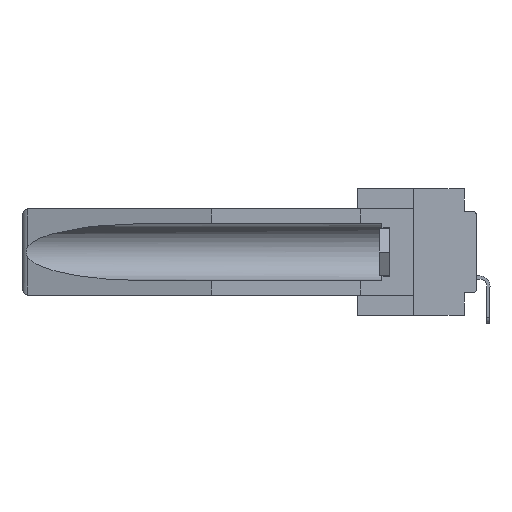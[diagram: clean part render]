
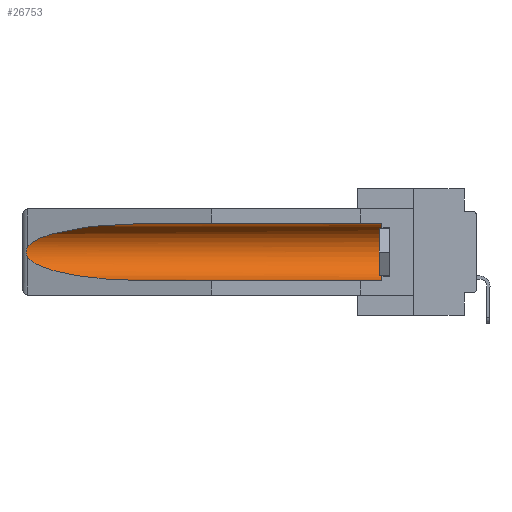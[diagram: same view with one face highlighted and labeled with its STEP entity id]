
A CAD part, left-side view. The second image highlights one B-rep face of the part: STEP entity #26753.
In plain terms, the highlighted cylindrical face has radius 2.857 mm (diameter 5.715 mm), a partial arc.
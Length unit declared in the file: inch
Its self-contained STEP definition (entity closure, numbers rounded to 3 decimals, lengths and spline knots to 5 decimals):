
#281 = VERTEX_POINT ( 'NONE', #3739 ) ;
#1954 = CARTESIAN_POINT ( 'NONE',  ( 0.2675, 1.53308, -0.17534 ) ) ;
#2335 = CARTESIAN_POINT ( 'NONE',  ( 0.2673, 1.53269, -0.17917 ) ) ;
#2608 = AXIS2_PLACEMENT_3D ( 'NONE', #23767, #16681, #25966 ) ;
#3291 = ORIENTED_EDGE ( 'NONE', *, *, #8695, .F. ) ;
#3420 = CARTESIAN_POINT ( 'NONE',  ( 0.26655, 1.53094, -0.18657 ) ) ;
#3661 = EDGE_CURVE ( 'NONE', #20136, #19773, #11870, .T. ) ;
#3739 = CARTESIAN_POINT ( 'NONE',  ( 0.155, 1.07973, -0.059 ) ) ;
#4217 = AXIS2_PLACEMENT_3D ( 'NONE', #11792, #9875, #16605 ) ;
#4889 = FACE_OUTER_BOUND ( 'NONE', #15215, .T. ) ;
#5228 = CARTESIAN_POINT ( 'NONE',  ( 0.2673, 1.5327, -0.16383 ) ) ;
#7863 = CARTESIAN_POINT ( 'NONE',  ( 0.26537, 1.52718, -0.14972 ) ) ;
#8695 = EDGE_CURVE ( 'NONE', #20136, #28436, #20644, .T. ) ;
#9158 = CARTESIAN_POINT ( 'NONE',  ( 0.21114, 1.30732, -0.284 ) ) ;
#9875 = DIRECTION ( 'NONE',  ( 0., 1., 0. ) ) ;
#10264 = CARTESIAN_POINT ( 'NONE',  ( 0.25451, 1.48313, -0.09465 ) ) ;
#11792 = CARTESIAN_POINT ( 'NONE',  ( 0.155, -0.30754, -0.1715 ) ) ;
#11870 = CIRCLE ( 'NONE', #2608, 0.1125 ) ;
#12776 = CARTESIAN_POINT ( 'NONE',  ( 0.155, 1.07973, -0.059 ) ) ;
#13152 = CARTESIAN_POINT ( 'NONE',  ( 0.2675, 1.53308, -0.16763 ) ) ;
#13375 = VECTOR ( 'NONE', #17002, 39.37008 ) ;
#13476 = CARTESIAN_POINT ( 'NONE',  ( 0.26537, 1.52718, -0.14972 ) ) ;
#13770 = CARTESIAN_POINT ( 'NONE',  ( 0.155, 0.126, -0.284 ) ) ;
#14582 = EDGE_CURVE ( 'NONE', #19773, #281, #29049, .T. ) ;
#15000 = CARTESIAN_POINT ( 'NONE',  ( 0.155, 0.126, -0.059 ) ) ;
#15215 = EDGE_LOOP ( 'NONE', ( #26105, #23425, #22288, #3291, #16965, #26800 ) ) ;
#15576 = EDGE_CURVE ( 'NONE', #22788, #28436, #26033, .T. ) ;
#15697 = CARTESIAN_POINT ( 'NONE',  ( 0.25451, 1.48313, -0.24835 ) ) ;
#16217 = CARTESIAN_POINT ( 'NONE',  ( 0.155, 1.07973, -0.284 ) ) ;
#16605 = DIRECTION ( 'NONE',  ( 0., 0., 1. ) ) ;
#16681 = DIRECTION ( 'NONE',  ( 0., -1., 0. ) ) ;
#16965 = ORIENTED_EDGE ( 'NONE', *, *, #3661, .T. ) ;
#17002 = DIRECTION ( 'NONE',  ( 0., 1., 0. ) ) ;
#17431 = EDGE_CURVE ( 'NONE', #281, #28802, #22397, .T. ) ;
#17567 = DIRECTION ( 'NONE',  ( 0., 1., 0. ) ) ;
#17605 = CARTESIAN_POINT ( 'NONE',  ( 0.26654, 1.53092, -0.15636 ) ) ;
#17902 = CARTESIAN_POINT ( 'NONE',  ( 0.155, 1.07973, -0.284 ) ) ;
#17921 = CARTESIAN_POINT ( 'NONE',  ( 0.26537, 1.52718, -0.14972 ) ) ;
#18101 = CARTESIAN_POINT ( 'NONE',  ( 0.26597, 1.52961, -0.15275 ) ) ;
#18341 = CARTESIAN_POINT ( 'NONE',  ( 0.26537, 1.52718, -0.19328 ) ) ;
#19763 = B_SPLINE_CURVE_WITH_KNOTS ( 'NONE', 3,
 ( #13476, #18101, #17605, #5228, #13152, #1954, #2335, #3420, #27256, #20576 ),
 .UNSPECIFIED., .F., .F.,
 ( 4, 2, 2, 2, 4 ),
 ( 0., 0.00029, 0.00058, 0.00087, 0.00117 ),
 .UNSPECIFIED. ) ;
#19773 = VERTEX_POINT ( 'NONE', #15000 ) ;
#20136 = VERTEX_POINT ( 'NONE', #13770 ) ;
#20576 = CARTESIAN_POINT ( 'NONE',  ( 0.26537, 1.52718, -0.19328 ) ) ;
#20644 = LINE ( 'NONE', #25984, #13375 ) ;
#22288 = ORIENTED_EDGE ( 'NONE', *, *, #15576, .T. ) ;
#22397 =( BOUNDED_CURVE ( )  B_SPLINE_CURVE ( 3, ( #12776, #26294, #10264, #7863 ),
 .UNSPECIFIED., .F., .F. ) 
 B_SPLINE_CURVE_WITH_KNOTS ( ( 4, 4 ),
 ( 4.71239, 6.08839 ),
 .UNSPECIFIED. ) 
 CURVE ( )  GEOMETRIC_REPRESENTATION_ITEM ( )  RATIONAL_B_SPLINE_CURVE ( ( 1., 0.848, 0.848, 1. ) ) 
 REPRESENTATION_ITEM ( '' )  );
#22788 = VERTEX_POINT ( 'NONE', #18341 ) ;
#23001 = VECTOR ( 'NONE', #17567, 39.37008 ) ;
#23425 = ORIENTED_EDGE ( 'NONE', *, *, #26706, .T. ) ;
#23767 = CARTESIAN_POINT ( 'NONE',  ( 0.155, 0.126, -0.1715 ) ) ;
#24352 = CYLINDRICAL_SURFACE ( 'NONE', #4217, 0.1125 ) ;
#24661 = CARTESIAN_POINT ( 'NONE',  ( 0.155, -0.30754, -0.059 ) ) ;
#25966 = DIRECTION ( 'NONE',  ( 0., 0., 1. ) ) ;
#25984 = CARTESIAN_POINT ( 'NONE',  ( 0.155, -0.30754, -0.284 ) ) ;
#26033 =( BOUNDED_CURVE ( )  B_SPLINE_CURVE ( 3, ( #27284, #15697, #9158, #17902 ),
 .UNSPECIFIED., .F., .F. ) 
 B_SPLINE_CURVE_WITH_KNOTS ( ( 4, 4 ),
 ( 0.1948, 1.5708 ),
 .UNSPECIFIED. ) 
 CURVE ( )  GEOMETRIC_REPRESENTATION_ITEM ( )  RATIONAL_B_SPLINE_CURVE ( ( 1., 0.848, 0.848, 1. ) ) 
 REPRESENTATION_ITEM ( '' )  );
#26105 = ORIENTED_EDGE ( 'NONE', *, *, #17431, .T. ) ;
#26294 = CARTESIAN_POINT ( 'NONE',  ( 0.21114, 1.30732, -0.059 ) ) ;
#26706 = EDGE_CURVE ( 'NONE', #28802, #22788, #19763, .T. ) ;
#26753 = ADVANCED_FACE ( 'NONE', ( #4889 ), #24352, .F. ) ;
#26800 = ORIENTED_EDGE ( 'NONE', *, *, #14582, .T. ) ;
#27256 = CARTESIAN_POINT ( 'NONE',  ( 0.26597, 1.5296, -0.19026 ) ) ;
#27284 = CARTESIAN_POINT ( 'NONE',  ( 0.26537, 1.52718, -0.19328 ) ) ;
#28436 = VERTEX_POINT ( 'NONE', #16217 ) ;
#28802 = VERTEX_POINT ( 'NONE', #17921 ) ;
#29049 = LINE ( 'NONE', #24661, #23001 ) ;
